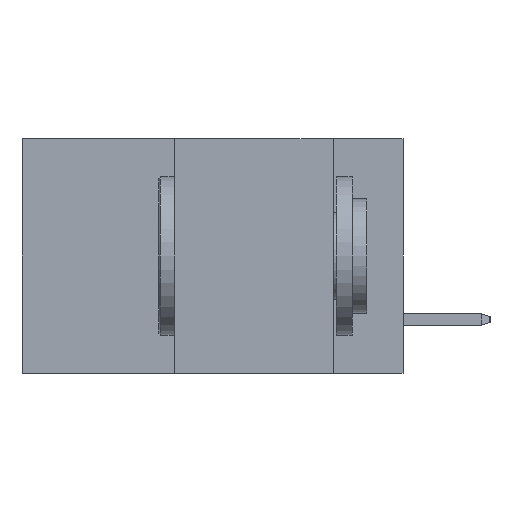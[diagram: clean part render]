
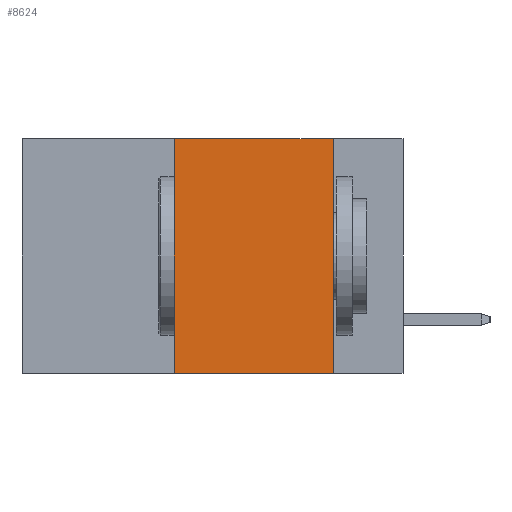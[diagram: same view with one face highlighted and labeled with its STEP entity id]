
A CAD part, left-side view. The second image highlights one B-rep face of the part: STEP entity #8624.
In plain terms, the highlighted planar face has unit normal (-1, 0, 0).
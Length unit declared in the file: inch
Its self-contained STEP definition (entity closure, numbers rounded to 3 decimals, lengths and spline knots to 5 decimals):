
#548 = LINE ( 'NONE', #5609, #9687 ) ;
#966 = CARTESIAN_POINT ( 'NONE',  ( 0., 0.6, 0. ) ) ;
#1076 = CARTESIAN_POINT ( 'NONE',  ( 0., 0.36, -0.37 ) ) ;
#1715 = CARTESIAN_POINT ( 'NONE',  ( 0., 0.6, -0.37 ) ) ;
#1880 = LINE ( 'NONE', #966, #9118 ) ;
#2236 = VERTEX_POINT ( 'NONE', #5461 ) ;
#2395 = VECTOR ( 'NONE', #5730, 39.37008 ) ;
#2419 = DIRECTION ( 'NONE',  ( 1., 0., 0. ) ) ;
#2498 = DIRECTION ( 'NONE',  ( 0., 0., -1. ) ) ;
#2945 = ORIENTED_EDGE ( 'NONE', *, *, #12009, .F. ) ;
#3408 = EDGE_CURVE ( 'NONE', #3490, #2236, #1880, .T. ) ;
#3490 = VERTEX_POINT ( 'NONE', #15154 ) ;
#4317 = LINE ( 'NONE', #4494, #2395 ) ;
#4494 = CARTESIAN_POINT ( 'NONE',  ( 0., 0.36, 0. ) ) ;
#5063 = EDGE_CURVE ( 'NONE', #2236, #14829, #548, .T. ) ;
#5461 = CARTESIAN_POINT ( 'NONE',  ( 0., 0.11, 0. ) ) ;
#5609 = CARTESIAN_POINT ( 'NONE',  ( 0., 0.11, 0. ) ) ;
#5730 = DIRECTION ( 'NONE',  ( 0., 0., 1. ) ) ;
#6122 = VERTEX_POINT ( 'NONE', #1076 ) ;
#6129 = VECTOR ( 'NONE', #9285, 39.37008 ) ;
#6961 = DIRECTION ( 'NONE',  ( 0., -1., 0. ) ) ;
#7560 = CARTESIAN_POINT ( 'NONE',  ( 0., 0.11, -0.37 ) ) ;
#7927 = ORIENTED_EDGE ( 'NONE', *, *, #5063, .F. ) ;
#8624 = ADVANCED_FACE ( 'NONE', ( #12729 ), #14049, .F. ) ;
#9118 = VECTOR ( 'NONE', #6961, 39.37008 ) ;
#9285 = DIRECTION ( 'NONE',  ( 0., -1., 0. ) ) ;
#9687 = VECTOR ( 'NONE', #12836, 39.37008 ) ;
#9746 = AXIS2_PLACEMENT_3D ( 'NONE', #10082, #2419, #2498 ) ;
#10082 = CARTESIAN_POINT ( 'NONE',  ( 0., 0.6, 0. ) ) ;
#10545 = LINE ( 'NONE', #1715, #6129 ) ;
#12009 = EDGE_CURVE ( 'NONE', #6122, #3490, #4317, .T. ) ;
#12509 = ORIENTED_EDGE ( 'NONE', *, *, #3408, .F. ) ;
#12589 = EDGE_CURVE ( 'NONE', #6122, #14829, #10545, .T. ) ;
#12729 = FACE_OUTER_BOUND ( 'NONE', #13236, .T. ) ;
#12836 = DIRECTION ( 'NONE',  ( 0., 0., -1. ) ) ;
#13236 = EDGE_LOOP ( 'NONE', ( #7927, #12509, #2945, #15183 ) ) ;
#14049 = PLANE ( 'NONE',  #9746 ) ;
#14829 = VERTEX_POINT ( 'NONE', #7560 ) ;
#15154 = CARTESIAN_POINT ( 'NONE',  ( 0., 0.36, 0. ) ) ;
#15183 = ORIENTED_EDGE ( 'NONE', *, *, #12589, .T. ) ;
